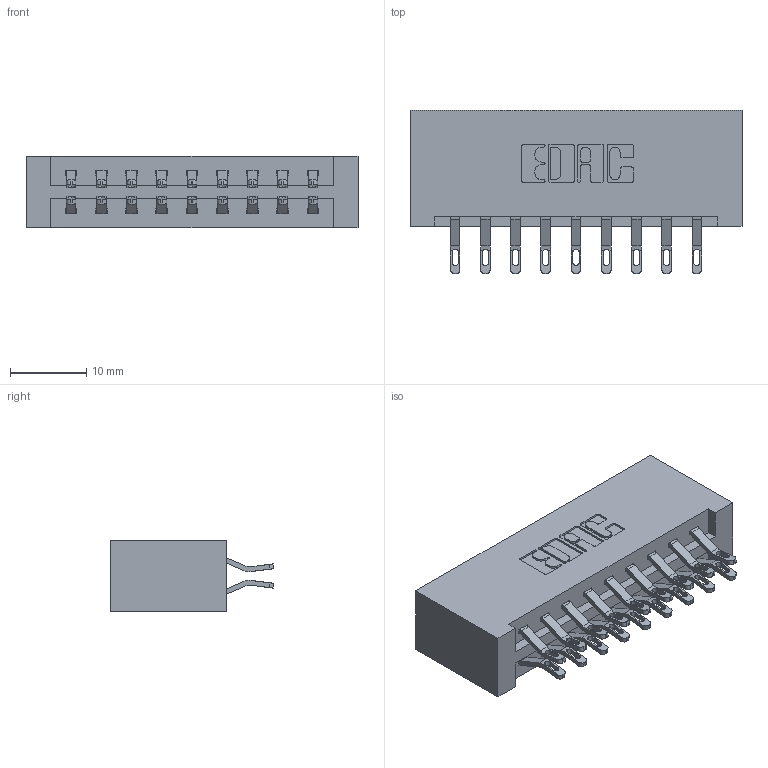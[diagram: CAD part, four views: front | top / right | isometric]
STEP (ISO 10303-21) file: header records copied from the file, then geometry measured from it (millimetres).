
FILE_DESCRIPTION (( 'STEP AP203' ), '1' );
FILE_NAME ('337-018-555-201.STEP', '2019-10-08T13:22:04', ( '' ), ( '' ), 'SwSTEP 2.0', 'SolidWorks 2016', '' );
FILE_SCHEMA (( 'CONFIG_CONTROL_DESIGN' ));
Length unit declared in the file: inch
Products named in the file (3): 337-018-555-201; 345-292-001_555 Tail; 337 Part_No Mounting Lugs
Assembly tree (19 placements, depth 2):
  337-018-555-201
    337 Part_No Mounting Lugs
    345-292-001_555 Tail  x18
Bounding box: 43.54 x 21.47 x 9.4 mm (x, y, z)
Volume: 4961.8 mm3; surface area: 5541.6 mm2
Topology: 19 solids, 19 shells, 1186 faces, 3689 edges, 2458 vertices
Faces by surface type: plane 714, cylinder 472
Entity records: 11295 total; most frequent: CARTESIAN_POINT 1964, ORIENTED_EDGE 1870, DIRECTION 1695, EDGE_CURVE 935, LINE 795, VECTOR 795, VERTEX_POINT 622, AXIS2_PLACEMENT_3D 450
